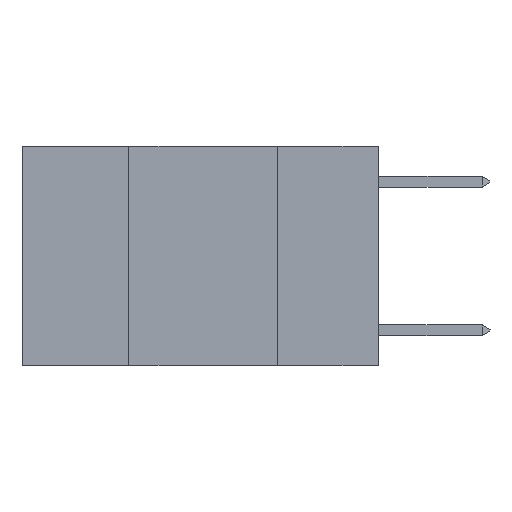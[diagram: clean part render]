
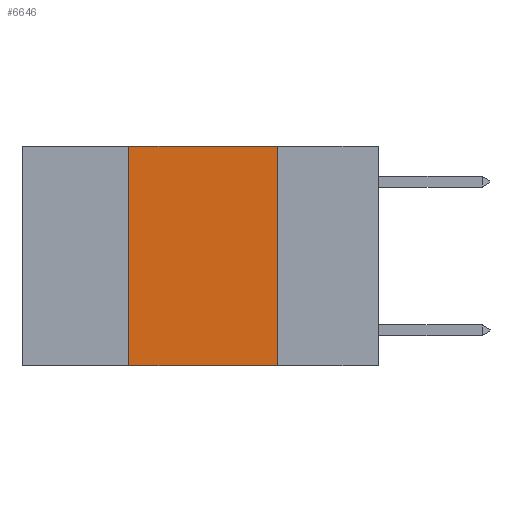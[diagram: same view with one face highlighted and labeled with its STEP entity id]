
A CAD part, left-side view. The second image highlights one B-rep face of the part: STEP entity #6646.
In plain terms, the highlighted planar face has unit normal (-1, 0, 0).
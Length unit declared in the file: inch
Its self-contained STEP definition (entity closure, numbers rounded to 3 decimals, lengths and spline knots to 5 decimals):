
#522 = DIRECTION ( 'NONE',  ( 1., 0., 0. ) ) ;
#689 = CARTESIAN_POINT ( 'NONE',  ( 0., 0.42, 0. ) ) ;
#977 = VECTOR ( 'NONE', #5575, 39.37008 ) ;
#1245 = LINE ( 'NONE', #7285, #977 ) ;
#1932 = EDGE_LOOP ( 'NONE', ( #5445, #7390, #9983, #10569 ) ) ;
#3198 = CARTESIAN_POINT ( 'NONE',  ( 0., 0.17, -0.37 ) ) ;
#3677 = VERTEX_POINT ( 'NONE', #4711 ) ;
#3880 = CARTESIAN_POINT ( 'NONE',  ( 0., 0.6, -0.37 ) ) ;
#3948 = VERTEX_POINT ( 'NONE', #6677 ) ;
#4089 = LINE ( 'NONE', #3880, #10596 ) ;
#4347 = EDGE_CURVE ( 'NONE', #3677, #9855, #9444, .T. ) ;
#4359 = EDGE_CURVE ( 'NONE', #3948, #6083, #11081, .T. ) ;
#4437 = EDGE_CURVE ( 'NONE', #3948, #9855, #4089, .T. ) ;
#4615 = CARTESIAN_POINT ( 'NONE',  ( 0., 0.17, 0. ) ) ;
#4641 = VECTOR ( 'NONE', #8081, 39.37008 ) ;
#4711 = CARTESIAN_POINT ( 'NONE',  ( 0., 0.17, 0. ) ) ;
#5016 = FACE_OUTER_BOUND ( 'NONE', #1932, .T. ) ;
#5445 = ORIENTED_EDGE ( 'NONE', *, *, #4347, .F. ) ;
#5575 = DIRECTION ( 'NONE',  ( 0., -1., 0. ) ) ;
#5802 = CARTESIAN_POINT ( 'NONE',  ( 0., 0.6, 0. ) ) ;
#6083 = VERTEX_POINT ( 'NONE', #689 ) ;
#6283 = AXIS2_PLACEMENT_3D ( 'NONE', #5802, #522, #6625 ) ;
#6625 = DIRECTION ( 'NONE',  ( 0., 0., -1. ) ) ;
#6646 = ADVANCED_FACE ( 'NONE', ( #5016 ), #7474, .F. ) ;
#6677 = CARTESIAN_POINT ( 'NONE',  ( 0., 0.42, -0.37 ) ) ;
#7224 = CARTESIAN_POINT ( 'NONE',  ( 0., 0.42, 0. ) ) ;
#7285 = CARTESIAN_POINT ( 'NONE',  ( 0., 0.6, 0. ) ) ;
#7390 = ORIENTED_EDGE ( 'NONE', *, *, #7969, .F. ) ;
#7474 = PLANE ( 'NONE',  #6283 ) ;
#7969 = EDGE_CURVE ( 'NONE', #6083, #3677, #1245, .T. ) ;
#8081 = DIRECTION ( 'NONE',  ( 0., 0., -1. ) ) ;
#8930 = VECTOR ( 'NONE', #10572, 39.37008 ) ;
#9023 = DIRECTION ( 'NONE',  ( 0., -1., 0. ) ) ;
#9444 = LINE ( 'NONE', #4615, #4641 ) ;
#9855 = VERTEX_POINT ( 'NONE', #3198 ) ;
#9983 = ORIENTED_EDGE ( 'NONE', *, *, #4359, .F. ) ;
#10569 = ORIENTED_EDGE ( 'NONE', *, *, #4437, .T. ) ;
#10572 = DIRECTION ( 'NONE',  ( 0., 0., 1. ) ) ;
#10596 = VECTOR ( 'NONE', #9023, 39.37008 ) ;
#11081 = LINE ( 'NONE', #7224, #8930 ) ;
